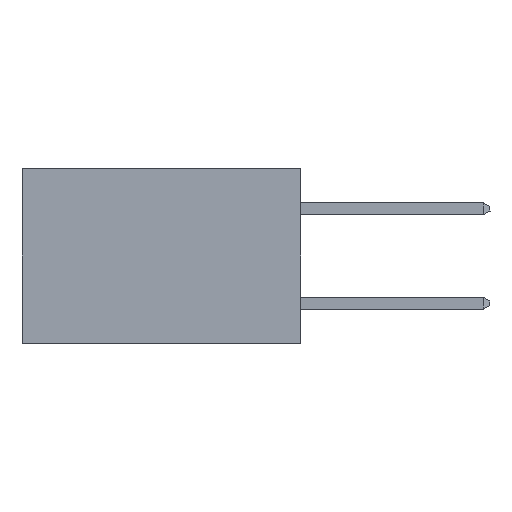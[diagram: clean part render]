
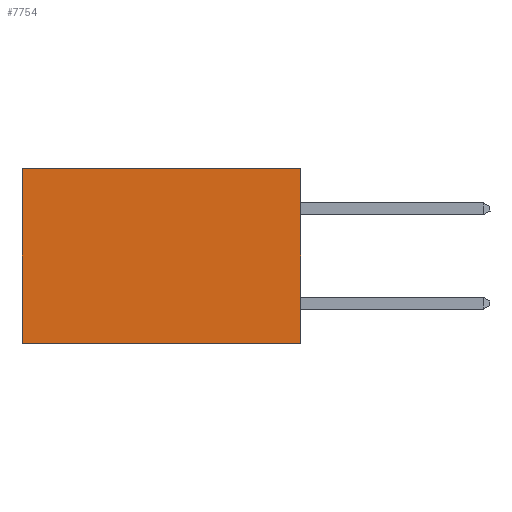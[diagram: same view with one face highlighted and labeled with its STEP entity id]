
A CAD part, left-side view. The second image highlights one B-rep face of the part: STEP entity #7754.
In plain terms, the highlighted planar face has unit normal (-1, 0, 0).
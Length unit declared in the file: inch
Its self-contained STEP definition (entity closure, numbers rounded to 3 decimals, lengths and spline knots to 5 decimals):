
#116 = VERTEX_POINT ( 'NONE', #13092 ) ;
#176 = CARTESIAN_POINT ( 'NONE',  ( 0.277, 0., 0. ) ) ;
#595 = DIRECTION ( 'NONE',  ( 0., 0., -1. ) ) ;
#806 = ORIENTED_EDGE ( 'NONE', *, *, #13375, .T. ) ;
#2030 = ORIENTED_EDGE ( 'NONE', *, *, #14426, .F. ) ;
#2557 = LINE ( 'NONE', #4742, #12927 ) ;
#2624 = VECTOR ( 'NONE', #16237, 39.37008 ) ;
#3469 = FACE_OUTER_BOUND ( 'NONE', #13061, .T. ) ;
#4601 = CARTESIAN_POINT ( 'NONE',  ( 0.277, 0., -0.37 ) ) ;
#4742 = CARTESIAN_POINT ( 'NONE',  ( 0.277, 0.59, -0.37 ) ) ;
#5244 = PLANE ( 'NONE',  #9582 ) ;
#6502 = DIRECTION ( 'NONE',  ( 1., 0., 0. ) ) ;
#6535 = ORIENTED_EDGE ( 'NONE', *, *, #14463, .F. ) ;
#7754 = ADVANCED_FACE ( 'NONE', ( #3469 ), #5244, .F. ) ;
#8432 = DIRECTION ( 'NONE',  ( 0., 0., -1. ) ) ;
#8996 = CARTESIAN_POINT ( 'NONE',  ( 0.277, 0.59, -0.37 ) ) ;
#9582 = AXIS2_PLACEMENT_3D ( 'NONE', #14241, #6502, #15522 ) ;
#9650 = CARTESIAN_POINT ( 'NONE',  ( 0.277, 0., -0.37 ) ) ;
#10265 = VECTOR ( 'NONE', #16081, 39.37008 ) ;
#10779 = VERTEX_POINT ( 'NONE', #8996 ) ;
#11081 = CARTESIAN_POINT ( 'NONE',  ( 0.277, 0., 0. ) ) ;
#11807 = EDGE_CURVE ( 'NONE', #14393, #116, #16334, .T. ) ;
#12927 = VECTOR ( 'NONE', #595, 39.37008 ) ;
#13061 = EDGE_LOOP ( 'NONE', ( #806, #2030, #6535, #16055 ) ) ;
#13092 = CARTESIAN_POINT ( 'NONE',  ( 0.277, 0.59, 0. ) ) ;
#13288 = LINE ( 'NONE', #4601, #16243 ) ;
#13375 = EDGE_CURVE ( 'NONE', #116, #10779, #2557, .T. ) ;
#13708 = LINE ( 'NONE', #9650, #10265 ) ;
#14081 = CARTESIAN_POINT ( 'NONE',  ( 0.277, 0., -0.37 ) ) ;
#14241 = CARTESIAN_POINT ( 'NONE',  ( 0.277, 0., -0.37 ) ) ;
#14393 = VERTEX_POINT ( 'NONE', #176 ) ;
#14426 = EDGE_CURVE ( 'NONE', #14628, #10779, #13708, .T. ) ;
#14463 = EDGE_CURVE ( 'NONE', #14393, #14628, #13288, .T. ) ;
#14628 = VERTEX_POINT ( 'NONE', #14081 ) ;
#15522 = DIRECTION ( 'NONE',  ( 0., 0., -1. ) ) ;
#16055 = ORIENTED_EDGE ( 'NONE', *, *, #11807, .T. ) ;
#16081 = DIRECTION ( 'NONE',  ( 0., 1., 0. ) ) ;
#16237 = DIRECTION ( 'NONE',  ( 0., 1., 0. ) ) ;
#16243 = VECTOR ( 'NONE', #8432, 39.37008 ) ;
#16334 = LINE ( 'NONE', #11081, #2624 ) ;
